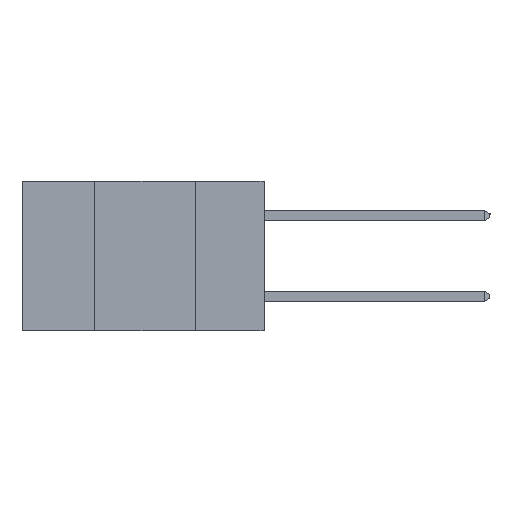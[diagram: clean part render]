
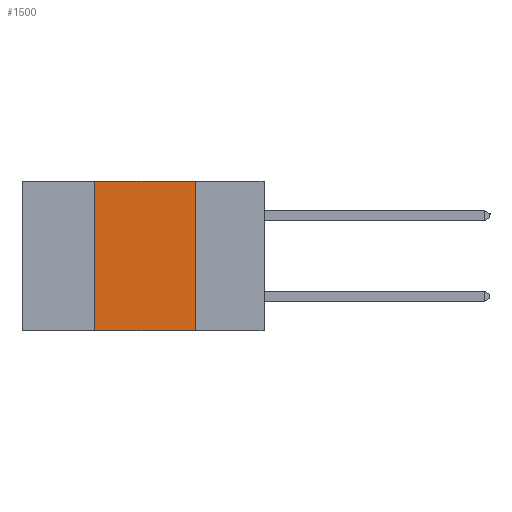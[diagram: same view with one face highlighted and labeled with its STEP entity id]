
A CAD part, left-side view. The second image highlights one B-rep face of the part: STEP entity #1500.
In plain terms, the highlighted planar face has unit normal (-1, 0, 0).
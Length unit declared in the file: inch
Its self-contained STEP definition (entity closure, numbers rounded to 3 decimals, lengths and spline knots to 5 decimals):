
#805 = VECTOR ( 'NONE', #3438, 39.37008 ) ;
#1100 = VECTOR ( 'NONE', #11907, 39.37008 ) ;
#1500 = ADVANCED_FACE ( 'NONE', ( #6643 ), #13936, .F. ) ;
#1690 = CARTESIAN_POINT ( 'NONE',  ( 0., 0.17, -0.37 ) ) ;
#1715 = VECTOR ( 'NONE', #3993, 39.37008 ) ;
#1985 = CARTESIAN_POINT ( 'NONE',  ( 0., 0.17, -0.37 ) ) ;
#2060 = ORIENTED_EDGE ( 'NONE', *, *, #21725, .F. ) ;
#2479 = CARTESIAN_POINT ( 'NONE',  ( 0., 0.6, 0. ) ) ;
#3120 = CARTESIAN_POINT ( 'NONE',  ( 0., 0.42, -0.37 ) ) ;
#3438 = DIRECTION ( 'NONE',  ( 0., -1., 0. ) ) ;
#3889 = CARTESIAN_POINT ( 'NONE',  ( 0., 0.42, -0.37 ) ) ;
#3921 = VERTEX_POINT ( 'NONE', #1985 ) ;
#3993 = DIRECTION ( 'NONE',  ( 0., 0., 1. ) ) ;
#4568 = EDGE_CURVE ( 'NONE', #11037, #3921, #19903, .T. ) ;
#5233 = DIRECTION ( 'NONE',  ( 1., 0., 0. ) ) ;
#5722 = ORIENTED_EDGE ( 'NONE', *, *, #7741, .T. ) ;
#6332 = VERTEX_POINT ( 'NONE', #12722 ) ;
#6534 = ORIENTED_EDGE ( 'NONE', *, *, #4568, .F. ) ;
#6643 = FACE_OUTER_BOUND ( 'NONE', #11984, .T. ) ;
#7636 = DIRECTION ( 'NONE',  ( 0., -1., 0. ) ) ;
#7741 = EDGE_CURVE ( 'NONE', #18624, #3921, #12152, .T. ) ;
#11037 = VERTEX_POINT ( 'NONE', #13135 ) ;
#11299 = ORIENTED_EDGE ( 'NONE', *, *, #11484, .F. ) ;
#11484 = EDGE_CURVE ( 'NONE', #6332, #11037, #13157, .T. ) ;
#11907 = DIRECTION ( 'NONE',  ( 0., 0., -1. ) ) ;
#11984 = EDGE_LOOP ( 'NONE', ( #6534, #11299, #2060, #5722 ) ) ;
#12152 = LINE ( 'NONE', #19100, #805 ) ;
#12235 = DIRECTION ( 'NONE',  ( 0., 0., -1. ) ) ;
#12593 = LINE ( 'NONE', #3889, #1715 ) ;
#12722 = CARTESIAN_POINT ( 'NONE',  ( 0., 0.42, 0. ) ) ;
#13135 = CARTESIAN_POINT ( 'NONE',  ( 0., 0.17, 0. ) ) ;
#13157 = LINE ( 'NONE', #2479, #18718 ) ;
#13936 = PLANE ( 'NONE',  #22214 ) ;
#18624 = VERTEX_POINT ( 'NONE', #3120 ) ;
#18718 = VECTOR ( 'NONE', #7636, 39.37008 ) ;
#19100 = CARTESIAN_POINT ( 'NONE',  ( 0., 0.6, -0.37 ) ) ;
#19903 = LINE ( 'NONE', #1690, #1100 ) ;
#20883 = CARTESIAN_POINT ( 'NONE',  ( 0., 0.6, 0. ) ) ;
#21725 = EDGE_CURVE ( 'NONE', #18624, #6332, #12593, .T. ) ;
#22214 = AXIS2_PLACEMENT_3D ( 'NONE', #20883, #5233, #12235 ) ;
